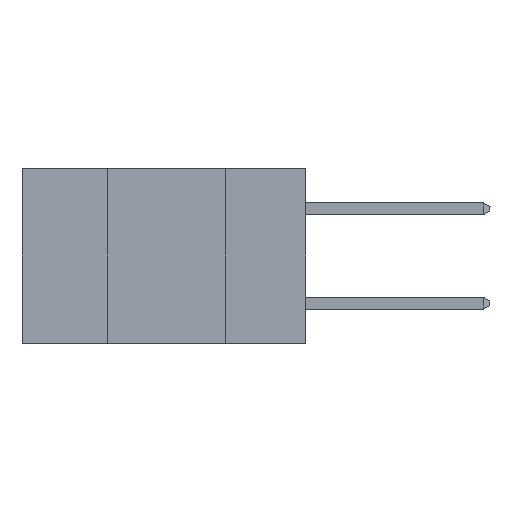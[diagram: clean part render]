
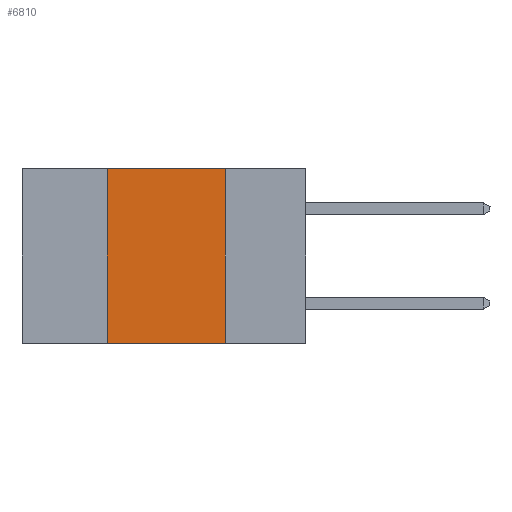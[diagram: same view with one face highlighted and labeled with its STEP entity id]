
A CAD part, left-side view. The second image highlights one B-rep face of the part: STEP entity #6810.
In plain terms, the highlighted planar face has unit normal (-1, 0, 0).
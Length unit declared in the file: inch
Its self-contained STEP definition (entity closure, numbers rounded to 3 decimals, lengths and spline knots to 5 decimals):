
#303 = PLANE ( 'NONE',  #26888 ) ;
#1200 = ORIENTED_EDGE ( 'NONE', *, *, #6906, .F. ) ;
#1320 = FACE_OUTER_BOUND ( 'NONE', #7684, .T. ) ;
#2034 = LINE ( 'NONE', #13309, #18335 ) ;
#2079 = VERTEX_POINT ( 'NONE', #21437 ) ;
#2300 = LINE ( 'NONE', #9470, #5677 ) ;
#2473 = EDGE_CURVE ( 'NONE', #5562, #18417, #2300, .T. ) ;
#3600 = DIRECTION ( 'NONE',  ( 0., -1., 0. ) ) ;
#5562 = VERTEX_POINT ( 'NONE', #23281 ) ;
#5677 = VECTOR ( 'NONE', #19742, 39.37008 ) ;
#5789 = VECTOR ( 'NONE', #6496, 39.37008 ) ;
#6496 = DIRECTION ( 'NONE',  ( 0., 0., -1. ) ) ;
#6810 = ADVANCED_FACE ( 'NONE', ( #1320 ), #303, .F. ) ;
#6906 = EDGE_CURVE ( 'NONE', #2079, #25532, #10755, .T. ) ;
#7684 = EDGE_LOOP ( 'NONE', ( #15215, #1200, #10338, #15769 ) ) ;
#9399 = CARTESIAN_POINT ( 'NONE',  ( 0., 0.17, 0. ) ) ;
#9470 = CARTESIAN_POINT ( 'NONE',  ( 0., 0.6, -0.37 ) ) ;
#9740 = VECTOR ( 'NONE', #3600, 39.37008 ) ;
#10338 = ORIENTED_EDGE ( 'NONE', *, *, #17574, .F. ) ;
#10755 = LINE ( 'NONE', #13639, #9740 ) ;
#13309 = CARTESIAN_POINT ( 'NONE',  ( 0., 0.42, 0. ) ) ;
#13499 = DIRECTION ( 'NONE',  ( 0., 0., 1. ) ) ;
#13639 = CARTESIAN_POINT ( 'NONE',  ( 0., 0.6, 0. ) ) ;
#14285 = LINE ( 'NONE', #9399, #5789 ) ;
#15215 = ORIENTED_EDGE ( 'NONE', *, *, #17289, .F. ) ;
#15444 = DIRECTION ( 'NONE',  ( 1., 0., 0. ) ) ;
#15769 = ORIENTED_EDGE ( 'NONE', *, *, #2473, .T. ) ;
#17289 = EDGE_CURVE ( 'NONE', #25532, #18417, #14285, .T. ) ;
#17574 = EDGE_CURVE ( 'NONE', #5562, #2079, #2034, .T. ) ;
#17732 = DIRECTION ( 'NONE',  ( 0., 0., -1. ) ) ;
#18335 = VECTOR ( 'NONE', #13499, 39.37008 ) ;
#18417 = VERTEX_POINT ( 'NONE', #18910 ) ;
#18910 = CARTESIAN_POINT ( 'NONE',  ( 0., 0.17, -0.37 ) ) ;
#19742 = DIRECTION ( 'NONE',  ( 0., -1., 0. ) ) ;
#19992 = CARTESIAN_POINT ( 'NONE',  ( 0., 0.6, 0. ) ) ;
#21437 = CARTESIAN_POINT ( 'NONE',  ( 0., 0.42, 0. ) ) ;
#23281 = CARTESIAN_POINT ( 'NONE',  ( 0., 0.42, -0.37 ) ) ;
#24503 = CARTESIAN_POINT ( 'NONE',  ( 0., 0.17, 0. ) ) ;
#25532 = VERTEX_POINT ( 'NONE', #24503 ) ;
#26888 = AXIS2_PLACEMENT_3D ( 'NONE', #19992, #15444, #17732 ) ;
